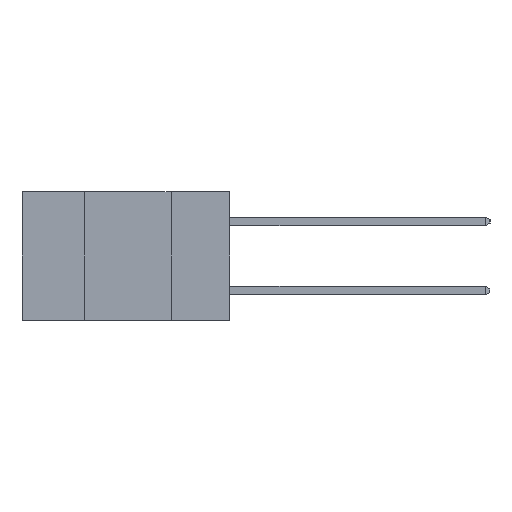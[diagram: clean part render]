
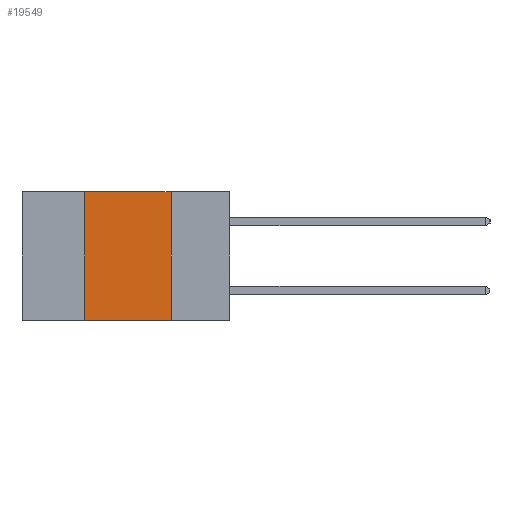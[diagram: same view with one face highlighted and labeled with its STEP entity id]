
A CAD part, left-side view. The second image highlights one B-rep face of the part: STEP entity #19549.
In plain terms, the highlighted planar face has unit normal (-1, 0, 0).
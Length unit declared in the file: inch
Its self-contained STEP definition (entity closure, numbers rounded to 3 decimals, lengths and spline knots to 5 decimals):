
#455 = CARTESIAN_POINT ( 'NONE',  ( 0., 0.42, -0.37 ) ) ;
#584 = DIRECTION ( 'NONE',  ( 0., -1., 0. ) ) ;
#2637 = CARTESIAN_POINT ( 'NONE',  ( 0., 0.42, 0. ) ) ;
#3413 = ORIENTED_EDGE ( 'NONE', *, *, #9906, .F. ) ;
#4043 = EDGE_CURVE ( 'NONE', #10622, #6312, #7193, .T. ) ;
#5033 = CARTESIAN_POINT ( 'NONE',  ( 0., 0.6, -0.37 ) ) ;
#6312 = VERTEX_POINT ( 'NONE', #10301 ) ;
#6383 = LINE ( 'NONE', #16321, #10293 ) ;
#6730 = DIRECTION ( 'NONE',  ( 0., -1., 0. ) ) ;
#7193 = LINE ( 'NONE', #8444, #16588 ) ;
#7748 = VERTEX_POINT ( 'NONE', #455 ) ;
#7915 = ORIENTED_EDGE ( 'NONE', *, *, #4043, .F. ) ;
#8444 = CARTESIAN_POINT ( 'NONE',  ( 0., 0.6, 0. ) ) ;
#8837 = DIRECTION ( 'NONE',  ( 1., 0., 0. ) ) ;
#9363 = CARTESIAN_POINT ( 'NONE',  ( 0., 0.17, -0.37 ) ) ;
#9906 = EDGE_CURVE ( 'NONE', #6312, #9923, #13181, .T. ) ;
#9923 = VERTEX_POINT ( 'NONE', #9363 ) ;
#10274 = AXIS2_PLACEMENT_3D ( 'NONE', #18775, #8837, #20393 ) ;
#10293 = VECTOR ( 'NONE', #17992, 39.37008 ) ;
#10301 = CARTESIAN_POINT ( 'NONE',  ( 0., 0.17, 0. ) ) ;
#10622 = VERTEX_POINT ( 'NONE', #2637 ) ;
#11110 = EDGE_LOOP ( 'NONE', ( #3413, #7915, #12824, #17264 ) ) ;
#12082 = PLANE ( 'NONE',  #10274 ) ;
#12824 = ORIENTED_EDGE ( 'NONE', *, *, #14366, .F. ) ;
#13181 = LINE ( 'NONE', #17646, #21448 ) ;
#14366 = EDGE_CURVE ( 'NONE', #7748, #10622, #6383, .T. ) ;
#14828 = VECTOR ( 'NONE', #6730, 39.37008 ) ;
#15358 = LINE ( 'NONE', #5033, #14828 ) ;
#16070 = FACE_OUTER_BOUND ( 'NONE', #11110, .T. ) ;
#16321 = CARTESIAN_POINT ( 'NONE',  ( 0., 0.42, 0. ) ) ;
#16588 = VECTOR ( 'NONE', #584, 39.37008 ) ;
#17264 = ORIENTED_EDGE ( 'NONE', *, *, #17424, .T. ) ;
#17424 = EDGE_CURVE ( 'NONE', #7748, #9923, #15358, .T. ) ;
#17646 = CARTESIAN_POINT ( 'NONE',  ( 0., 0.17, 0. ) ) ;
#17992 = DIRECTION ( 'NONE',  ( 0., 0., 1. ) ) ;
#18775 = CARTESIAN_POINT ( 'NONE',  ( 0., 0.6, 0. ) ) ;
#19282 = DIRECTION ( 'NONE',  ( 0., 0., -1. ) ) ;
#19549 = ADVANCED_FACE ( 'NONE', ( #16070 ), #12082, .F. ) ;
#20393 = DIRECTION ( 'NONE',  ( 0., 0., -1. ) ) ;
#21448 = VECTOR ( 'NONE', #19282, 39.37008 ) ;
